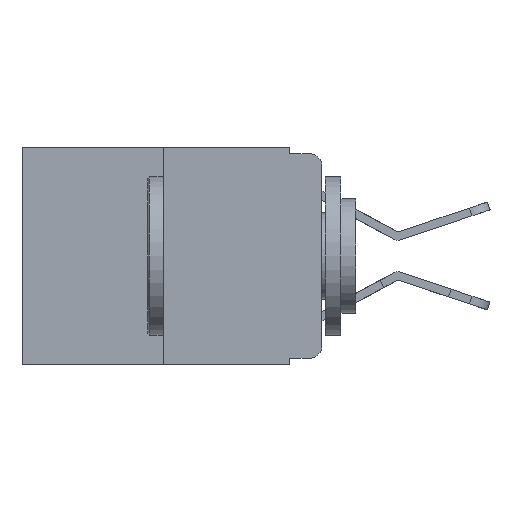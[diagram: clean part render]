
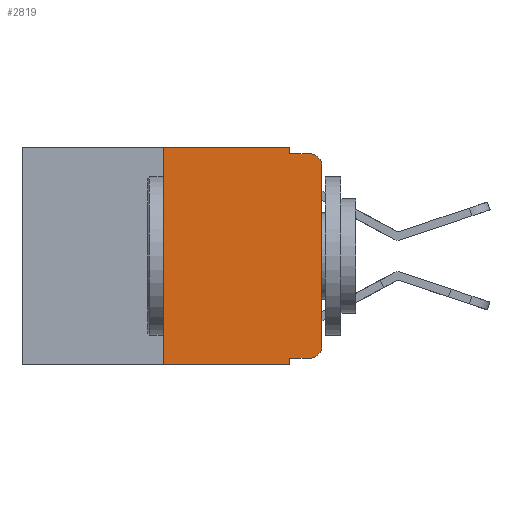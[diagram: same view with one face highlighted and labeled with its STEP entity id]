
A CAD part, left-side view. The second image highlights one B-rep face of the part: STEP entity #2819.
In plain terms, the highlighted planar face has unit normal (-1, 0, 0).
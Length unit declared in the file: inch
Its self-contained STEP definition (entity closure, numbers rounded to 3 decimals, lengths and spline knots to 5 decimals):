
#35 = DIRECTION ( 'NONE',  ( 0., -1., 0. ) ) ;
#74 = DIRECTION ( 'NONE',  ( 0., -1., 0. ) ) ;
#207 = CARTESIAN_POINT ( 'NONE',  ( 0., 0.051, -0.343 ) ) ;
#661 = DIRECTION ( 'NONE',  ( 0., 0., 1. ) ) ;
#807 = EDGE_CURVE ( 'NONE', #4808, #20818, #19888, .T. ) ;
#1043 = EDGE_LOOP ( 'NONE', ( #12692, #9770, #22594, #3069, #21999, #12416, #23257, #8202, #27035, #16814 ) ) ;
#1112 = AXIS2_PLACEMENT_3D ( 'NONE', #25099, #18976, #12463 ) ;
#1592 = VECTOR ( 'NONE', #25106, 39.37008 ) ;
#1619 = VECTOR ( 'NONE', #35, 39.37008 ) ;
#1724 = DIRECTION ( 'NONE',  ( -1., 0., 0. ) ) ;
#1786 = CARTESIAN_POINT ( 'NONE',  ( 0., 0.02, -0.313 ) ) ;
#1988 = CARTESIAN_POINT ( 'NONE',  ( 0., 0.051, 0. ) ) ;
#2261 = VERTEX_POINT ( 'NONE', #4687 ) ;
#2329 = CARTESIAN_POINT ( 'NONE',  ( 0., 0.473, 0. ) ) ;
#2454 = FACE_OUTER_BOUND ( 'NONE', #1043, .T. ) ;
#2563 = VERTEX_POINT ( 'NONE', #207 ) ;
#2660 = LINE ( 'NONE', #13474, #13937 ) ;
#2753 = VECTOR ( 'NONE', #19049, 39.37008 ) ;
#2783 = EDGE_CURVE ( 'NONE', #5899, #13194, #25210, .T. ) ;
#2819 = ADVANCED_FACE ( 'NONE', ( #2454 ), #25704, .F. ) ;
#3069 = ORIENTED_EDGE ( 'NONE', *, *, #2783, .F. ) ;
#3098 = CARTESIAN_POINT ( 'NONE',  ( 0., 0.02, -0.01 ) ) ;
#3193 = CARTESIAN_POINT ( 'NONE',  ( 0., 0.051, 0. ) ) ;
#3476 = DIRECTION ( 'NONE',  ( 0., 0., -1. ) ) ;
#4084 = VERTEX_POINT ( 'NONE', #20350 ) ;
#4364 = EDGE_CURVE ( 'NONE', #4911, #2563, #8541, .T. ) ;
#4537 = EDGE_CURVE ( 'NONE', #16404, #25175, #26414, .T. ) ;
#4687 = CARTESIAN_POINT ( 'NONE',  ( 0., 0.25, -0.343 ) ) ;
#4808 = VERTEX_POINT ( 'NONE', #6425 ) ;
#4911 = VERTEX_POINT ( 'NONE', #14955 ) ;
#5632 = EDGE_CURVE ( 'NONE', #13194, #25175, #7501, .T. ) ;
#5899 = VERTEX_POINT ( 'NONE', #3193 ) ;
#6425 = CARTESIAN_POINT ( 'NONE',  ( 0., 0.02, -0.333 ) ) ;
#6811 = EDGE_CURVE ( 'NONE', #4911, #4808, #24708, .T. ) ;
#7501 = LINE ( 'NONE', #25110, #1619 ) ;
#8086 = CARTESIAN_POINT ( 'NONE',  ( 0., 0.051, -0.333 ) ) ;
#8202 = ORIENTED_EDGE ( 'NONE', *, *, #4364, .F. ) ;
#8371 = CARTESIAN_POINT ( 'NONE',  ( 0., 0.051, -0.01 ) ) ;
#8541 = LINE ( 'NONE', #23114, #2753 ) ;
#9770 = ORIENTED_EDGE ( 'NONE', *, *, #4537, .T. ) ;
#10917 = CARTESIAN_POINT ( 'NONE',  ( 0., 0.473, -0.343 ) ) ;
#11302 = VECTOR ( 'NONE', #24442, 39.37008 ) ;
#11402 = DIRECTION ( 'NONE',  ( -1., 0., 0. ) ) ;
#12416 = ORIENTED_EDGE ( 'NONE', *, *, #24106, .F. ) ;
#12463 = DIRECTION ( 'NONE',  ( 0., 0., -1. ) ) ;
#12692 = ORIENTED_EDGE ( 'NONE', *, *, #26795, .T. ) ;
#13006 = DIRECTION ( 'NONE',  ( 0., -1., 0. ) ) ;
#13073 = DIRECTION ( 'NONE',  ( 0., 0., -1. ) ) ;
#13194 = VERTEX_POINT ( 'NONE', #8371 ) ;
#13474 = CARTESIAN_POINT ( 'NONE',  ( 0., 0.25, 0. ) ) ;
#13937 = VECTOR ( 'NONE', #661, 39.37008 ) ;
#14776 = AXIS2_PLACEMENT_3D ( 'NONE', #1786, #1724, #3476 ) ;
#14955 = CARTESIAN_POINT ( 'NONE',  ( 0., 0.051, -0.333 ) ) ;
#15432 = CARTESIAN_POINT ( 'NONE',  ( 0., 0., -0.03 ) ) ;
#15884 = LINE ( 'NONE', #2329, #26100 ) ;
#16404 = VERTEX_POINT ( 'NONE', #15432 ) ;
#16814 = ORIENTED_EDGE ( 'NONE', *, *, #807, .T. ) ;
#17972 = EDGE_CURVE ( 'NONE', #4084, #5899, #15884, .T. ) ;
#18976 = DIRECTION ( 'NONE',  ( 1., 0., 0. ) ) ;
#19049 = DIRECTION ( 'NONE',  ( 0., 0., -1. ) ) ;
#19790 = VECTOR ( 'NONE', #13073, 39.37008 ) ;
#19888 = CIRCLE ( 'NONE', #14776, 0.02 ) ;
#20038 = LINE ( 'NONE', #10917, #24813 ) ;
#20350 = CARTESIAN_POINT ( 'NONE',  ( 0., 0.25, 0. ) ) ;
#20818 = VERTEX_POINT ( 'NONE', #21422 ) ;
#21422 = CARTESIAN_POINT ( 'NONE',  ( 0., 0., -0.313 ) ) ;
#21999 = ORIENTED_EDGE ( 'NONE', *, *, #17972, .F. ) ;
#22594 = ORIENTED_EDGE ( 'NONE', *, *, #5632, .F. ) ;
#23094 = CARTESIAN_POINT ( 'NONE',  ( 0., 0., 0. ) ) ;
#23114 = CARTESIAN_POINT ( 'NONE',  ( 0., 0.051, 0. ) ) ;
#23257 = ORIENTED_EDGE ( 'NONE', *, *, #24943, .T. ) ;
#23651 = CARTESIAN_POINT ( 'NONE',  ( 0., 0.02, -0.03 ) ) ;
#24106 = EDGE_CURVE ( 'NONE', #2261, #4084, #2660, .T. ) ;
#24240 = AXIS2_PLACEMENT_3D ( 'NONE', #23651, #11402, #25652 ) ;
#24436 = LINE ( 'NONE', #23094, #1592 ) ;
#24442 = DIRECTION ( 'NONE',  ( 0., -1., 0. ) ) ;
#24708 = LINE ( 'NONE', #8086, #11302 ) ;
#24813 = VECTOR ( 'NONE', #13006, 39.37008 ) ;
#24943 = EDGE_CURVE ( 'NONE', #2261, #2563, #20038, .T. ) ;
#25099 = CARTESIAN_POINT ( 'NONE',  ( 0., 0.473, 0. ) ) ;
#25106 = DIRECTION ( 'NONE',  ( 0., 0., 1. ) ) ;
#25110 = CARTESIAN_POINT ( 'NONE',  ( 0., 0.051, -0.01 ) ) ;
#25175 = VERTEX_POINT ( 'NONE', #3098 ) ;
#25210 = LINE ( 'NONE', #1988, #19790 ) ;
#25652 = DIRECTION ( 'NONE',  ( 0., 0., -1. ) ) ;
#25704 = PLANE ( 'NONE',  #1112 ) ;
#26100 = VECTOR ( 'NONE', #74, 39.37008 ) ;
#26414 = CIRCLE ( 'NONE', #24240, 0.02 ) ;
#26795 = EDGE_CURVE ( 'NONE', #20818, #16404, #24436, .T. ) ;
#27035 = ORIENTED_EDGE ( 'NONE', *, *, #6811, .T. ) ;
